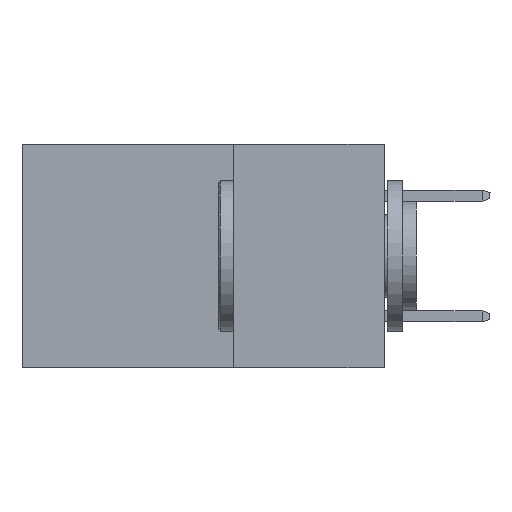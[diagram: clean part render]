
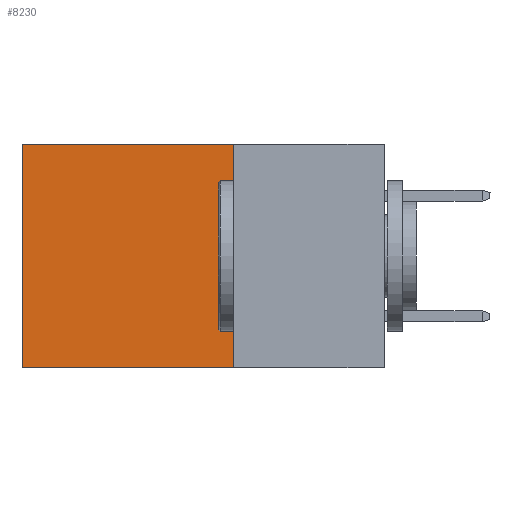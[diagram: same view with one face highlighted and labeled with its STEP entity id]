
A CAD part, left-side view. The second image highlights one B-rep face of the part: STEP entity #8230.
In plain terms, the highlighted planar face has unit normal (-1, 0, 0).
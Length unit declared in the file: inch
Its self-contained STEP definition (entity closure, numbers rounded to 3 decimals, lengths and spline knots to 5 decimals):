
#314 = DIRECTION ( 'NONE',  ( 1., 0., 0. ) ) ;
#1698 = VECTOR ( 'NONE', #20714, 39.37008 ) ;
#1898 = VECTOR ( 'NONE', #29616, 39.37008 ) ;
#2069 = LINE ( 'NONE', #17718, #8263 ) ;
#5193 = CARTESIAN_POINT ( 'NONE',  ( 0.298, 0.25, -0.37 ) ) ;
#5564 = EDGE_LOOP ( 'NONE', ( #14197, #16432, #23457, #23212 ) ) ;
#6491 = VECTOR ( 'NONE', #7851, 39.37008 ) ;
#6556 = CARTESIAN_POINT ( 'NONE',  ( 0.298, 0.25, 0. ) ) ;
#7020 = VERTEX_POINT ( 'NONE', #9039 ) ;
#7344 = DIRECTION ( 'NONE',  ( 0., 0., -1. ) ) ;
#7714 = VERTEX_POINT ( 'NONE', #19409 ) ;
#7851 = DIRECTION ( 'NONE',  ( 0., 1., 0. ) ) ;
#8165 = PLANE ( 'NONE',  #23044 ) ;
#8230 = ADVANCED_FACE ( 'NONE', ( #28972 ), #8165, .F. ) ;
#8263 = VECTOR ( 'NONE', #7344, 39.37008 ) ;
#8348 = CARTESIAN_POINT ( 'NONE',  ( 0.298, 0.25, -0.37 ) ) ;
#9039 = CARTESIAN_POINT ( 'NONE',  ( 0.298, 0.6, 0. ) ) ;
#9347 = EDGE_CURVE ( 'NONE', #7714, #13725, #23402, .T. ) ;
#13036 = CARTESIAN_POINT ( 'NONE',  ( 0.298, 0.6, -0.37 ) ) ;
#13401 = EDGE_CURVE ( 'NONE', #7020, #14142, #2069, .T. ) ;
#13725 = VERTEX_POINT ( 'NONE', #8348 ) ;
#14142 = VERTEX_POINT ( 'NONE', #13036 ) ;
#14197 = ORIENTED_EDGE ( 'NONE', *, *, #13401, .T. ) ;
#14790 = EDGE_CURVE ( 'NONE', #7714, #7020, #22409, .T. ) ;
#16033 = CARTESIAN_POINT ( 'NONE',  ( 0.298, 0.25, 0. ) ) ;
#16432 = ORIENTED_EDGE ( 'NONE', *, *, #23568, .F. ) ;
#17718 = CARTESIAN_POINT ( 'NONE',  ( 0.298, 0.6, 0. ) ) ;
#18627 = DIRECTION ( 'NONE',  ( 0., 0., -1. ) ) ;
#19409 = CARTESIAN_POINT ( 'NONE',  ( 0.298, 0.25, 0. ) ) ;
#20714 = DIRECTION ( 'NONE',  ( 0., 1., 0. ) ) ;
#22409 = LINE ( 'NONE', #33260, #1698 ) ;
#23044 = AXIS2_PLACEMENT_3D ( 'NONE', #16033, #314, #18627 ) ;
#23212 = ORIENTED_EDGE ( 'NONE', *, *, #14790, .T. ) ;
#23402 = LINE ( 'NONE', #6556, #1898 ) ;
#23457 = ORIENTED_EDGE ( 'NONE', *, *, #9347, .F. ) ;
#23568 = EDGE_CURVE ( 'NONE', #13725, #14142, #26965, .T. ) ;
#26965 = LINE ( 'NONE', #5193, #6491 ) ;
#28972 = FACE_OUTER_BOUND ( 'NONE', #5564, .T. ) ;
#29616 = DIRECTION ( 'NONE',  ( 0., 0., -1. ) ) ;
#33260 = CARTESIAN_POINT ( 'NONE',  ( 0.298, 0.25, 0. ) ) ;
